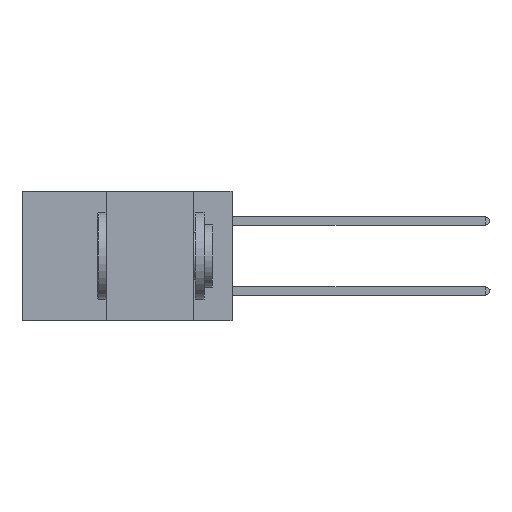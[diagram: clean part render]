
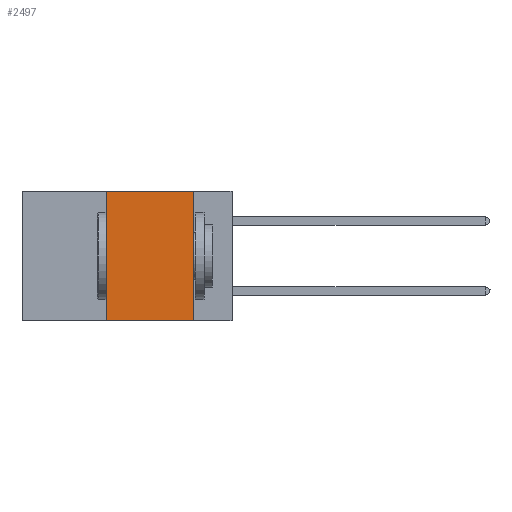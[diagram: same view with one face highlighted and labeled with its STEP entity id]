
A CAD part, left-side view. The second image highlights one B-rep face of the part: STEP entity #2497.
In plain terms, the highlighted planar face has unit normal (-1, 0, 0).
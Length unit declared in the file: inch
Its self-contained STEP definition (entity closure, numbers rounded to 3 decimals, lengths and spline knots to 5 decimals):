
#2497 = ADVANCED_FACE ( 'NONE', ( #23433 ), #9555, .F. ) ;
#4674 = EDGE_CURVE ( 'NONE', #17805, #26937, #23313, .T. ) ;
#4791 = ORIENTED_EDGE ( 'NONE', *, *, #25708, .F. ) ;
#4819 = VERTEX_POINT ( 'NONE', #14347 ) ;
#4912 = LINE ( 'NONE', #18189, #5909 ) ;
#5275 = CARTESIAN_POINT ( 'NONE',  ( 0., 0.11, 0. ) ) ;
#5909 = VECTOR ( 'NONE', #9373, 39.37008 ) ;
#6411 = CARTESIAN_POINT ( 'NONE',  ( 0., 0.6, -0.37 ) ) ;
#7559 = CARTESIAN_POINT ( 'NONE',  ( 0., 0.36, 0. ) ) ;
#8715 = VECTOR ( 'NONE', #21439, 39.37008 ) ;
#9373 = DIRECTION ( 'NONE',  ( 0., 0., -1. ) ) ;
#9555 = PLANE ( 'NONE',  #13851 ) ;
#10181 = EDGE_CURVE ( 'NONE', #21779, #4819, #4912, .T. ) ;
#10195 = VECTOR ( 'NONE', #11925, 39.37008 ) ;
#11434 = EDGE_LOOP ( 'NONE', ( #17284, #4791, #26054, #21302 ) ) ;
#11925 = DIRECTION ( 'NONE',  ( 0., 0., 1. ) ) ;
#13851 = AXIS2_PLACEMENT_3D ( 'NONE', #24577, #24482, #18197 ) ;
#14347 = CARTESIAN_POINT ( 'NONE',  ( 0., 0.11, -0.37 ) ) ;
#17284 = ORIENTED_EDGE ( 'NONE', *, *, #10181, .F. ) ;
#17805 = VERTEX_POINT ( 'NONE', #25269 ) ;
#18189 = CARTESIAN_POINT ( 'NONE',  ( 0., 0.11, 0. ) ) ;
#18197 = DIRECTION ( 'NONE',  ( 0., 0., -1. ) ) ;
#18253 = CARTESIAN_POINT ( 'NONE',  ( 0., 0.36, 0. ) ) ;
#19114 = DIRECTION ( 'NONE',  ( 0., -1., 0. ) ) ;
#19266 = LINE ( 'NONE', #6411, #19931 ) ;
#19931 = VECTOR ( 'NONE', #19114, 39.37008 ) ;
#21302 = ORIENTED_EDGE ( 'NONE', *, *, #21952, .T. ) ;
#21439 = DIRECTION ( 'NONE',  ( 0., -1., 0. ) ) ;
#21779 = VERTEX_POINT ( 'NONE', #5275 ) ;
#21952 = EDGE_CURVE ( 'NONE', #17805, #4819, #19266, .T. ) ;
#23313 = LINE ( 'NONE', #7559, #10195 ) ;
#23433 = FACE_OUTER_BOUND ( 'NONE', #11434, .T. ) ;
#24482 = DIRECTION ( 'NONE',  ( 1., 0., 0. ) ) ;
#24577 = CARTESIAN_POINT ( 'NONE',  ( 0., 0.6, 0. ) ) ;
#25269 = CARTESIAN_POINT ( 'NONE',  ( 0., 0.36, -0.37 ) ) ;
#25563 = CARTESIAN_POINT ( 'NONE',  ( 0., 0.6, 0. ) ) ;
#25708 = EDGE_CURVE ( 'NONE', #26937, #21779, #25846, .T. ) ;
#25846 = LINE ( 'NONE', #25563, #8715 ) ;
#26054 = ORIENTED_EDGE ( 'NONE', *, *, #4674, .F. ) ;
#26937 = VERTEX_POINT ( 'NONE', #18253 ) ;
